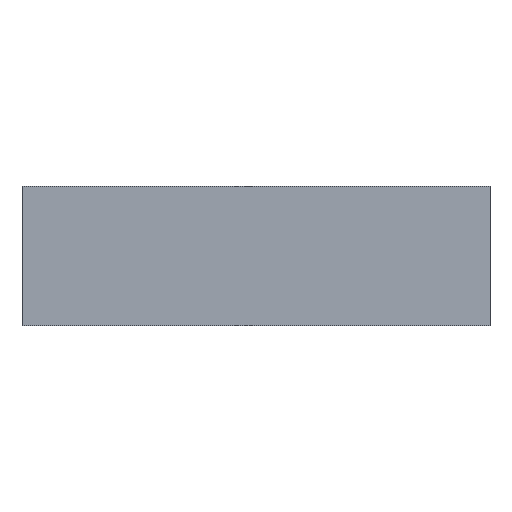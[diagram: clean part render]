
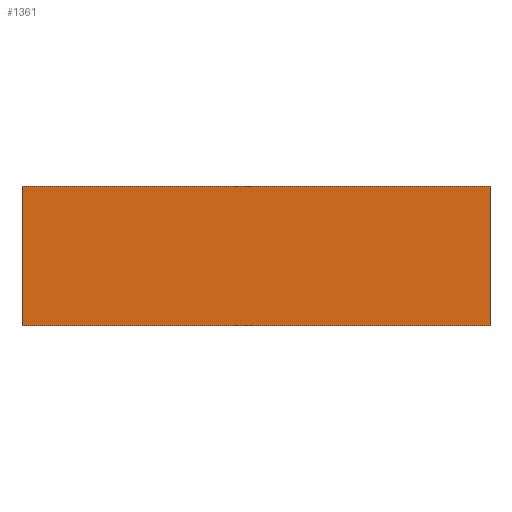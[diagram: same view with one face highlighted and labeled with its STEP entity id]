
A CAD part, front view. The second image highlights one B-rep face of the part: STEP entity #1361.
In plain terms, the highlighted planar face has unit normal (0, -1, 0).
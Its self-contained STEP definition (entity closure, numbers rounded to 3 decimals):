
#3 = CARTESIAN_POINT ( 'NONE',  ( -25.2, -50.325, 15. ) ) ;
#9 = VERTEX_POINT ( 'NONE', #76 ) ;
#24 = VERTEX_POINT ( 'NONE', #180 ) ;
#25 = ORIENTED_EDGE ( 'NONE', *, *, #1076, .T. ) ;
#43 = EDGE_CURVE ( 'NONE', #9, #1288, #859, .T. ) ;
#76 = CARTESIAN_POINT ( 'NONE',  ( -25.2, -50.325, 15. ) ) ;
#94 = CARTESIAN_POINT ( 'NONE',  ( -25.2, -50.325, 15. ) ) ;
#115 = LINE ( 'NONE', #94, #302 ) ;
#116 = EDGE_CURVE ( 'NONE', #9, #1402, #115, .T. ) ;
#137 = CARTESIAN_POINT ( 'NONE',  ( 25.2, -50.325, 15. ) ) ;
#169 = LINE ( 'NONE', #137, #1098 ) ;
#180 = CARTESIAN_POINT ( 'NONE',  ( 25.2, -50.325, 0. ) ) ;
#203 = DIRECTION ( 'NONE',  ( 1., 0., 0. ) ) ;
#282 = VECTOR ( 'NONE', #1256, 1000. ) ;
#302 = VECTOR ( 'NONE', #203, 1000. ) ;
#372 = AXIS2_PLACEMENT_3D ( 'NONE', #3, #441, #773 ) ;
#374 = EDGE_CURVE ( 'NONE', #1402, #24, #169, .T. ) ;
#407 = CARTESIAN_POINT ( 'NONE',  ( -25.2, -50.325, 0. ) ) ;
#433 = CARTESIAN_POINT ( 'NONE',  ( 25.2, -50.325, 15. ) ) ;
#441 = DIRECTION ( 'NONE',  ( 0., 1., 0. ) ) ;
#704 = LINE ( 'NONE', #1058, #282 ) ;
#773 = DIRECTION ( 'NONE',  ( 0., 0., 1. ) ) ;
#848 = CARTESIAN_POINT ( 'NONE',  ( -25.2, -50.325, 15. ) ) ;
#859 = LINE ( 'NONE', #848, #1233 ) ;
#878 = ORIENTED_EDGE ( 'NONE', *, *, #374, .F. ) ;
#901 = DIRECTION ( 'NONE',  ( 0., 0., -1. ) ) ;
#996 = EDGE_LOOP ( 'NONE', ( #25, #878, #1004, #1287 ) ) ;
#1004 = ORIENTED_EDGE ( 'NONE', *, *, #116, .F. ) ;
#1047 = FACE_OUTER_BOUND ( 'NONE', #996, .T. ) ;
#1058 = CARTESIAN_POINT ( 'NONE',  ( -25.2, -50.325, 0. ) ) ;
#1076 = EDGE_CURVE ( 'NONE', #1288, #24, #704, .T. ) ;
#1098 = VECTOR ( 'NONE', #901, 1000. ) ;
#1233 = VECTOR ( 'NONE', #1274, 1000. ) ;
#1256 = DIRECTION ( 'NONE',  ( 1., 0., 0. ) ) ;
#1274 = DIRECTION ( 'NONE',  ( 0., 0., -1. ) ) ;
#1287 = ORIENTED_EDGE ( 'NONE', *, *, #43, .T. ) ;
#1288 = VERTEX_POINT ( 'NONE', #407 ) ;
#1361 = ADVANCED_FACE ( 'NONE', ( #1047 ), #1425, .F. ) ;
#1402 = VERTEX_POINT ( 'NONE', #433 ) ;
#1425 = PLANE ( 'NONE',  #372 ) ;
